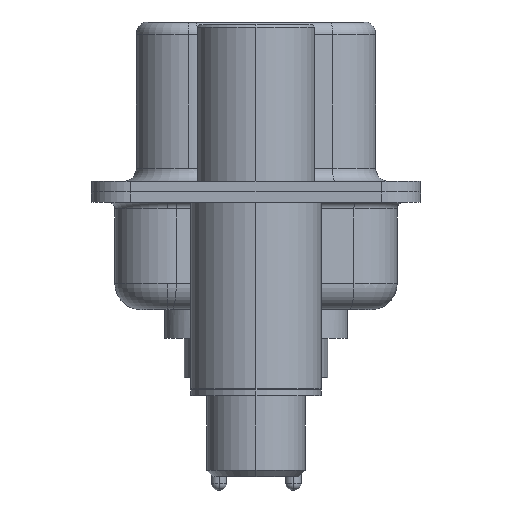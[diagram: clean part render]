
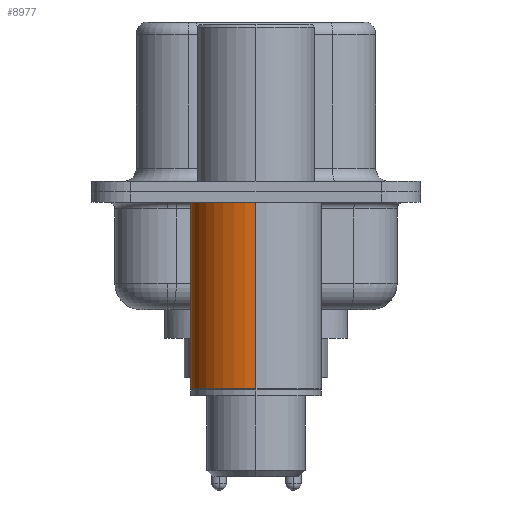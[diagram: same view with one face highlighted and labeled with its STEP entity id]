
A CAD part, left-side view. The second image highlights one B-rep face of the part: STEP entity #8977.
In plain terms, the highlighted cylindrical face has radius 2.5 mm (diameter 5 mm), a partial arc.
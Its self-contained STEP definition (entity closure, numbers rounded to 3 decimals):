
#102 = DIRECTION ( 'NONE',  ( 0., 0., 1. ) ) ;
#384 = CYLINDRICAL_SURFACE ( 'NONE', #8981, 2.5 ) ;
#977 = CARTESIAN_POINT ( 'NONE',  ( 2.5, 0., -0.4 ) ) ;
#1203 = DIRECTION ( 'NONE',  ( 1., 0., 0. ) ) ;
#2478 = EDGE_CURVE ( 'NONE', #8512, #4601, #16579, .T. ) ;
#2485 = ORIENTED_EDGE ( 'NONE', *, *, #2478, .F. ) ;
#2746 = DIRECTION ( 'NONE',  ( 0., 0., 1. ) ) ;
#3062 = DIRECTION ( 'NONE',  ( 0., 0., 1. ) ) ;
#3066 = LINE ( 'NONE', #19043, #12439 ) ;
#3137 = CARTESIAN_POINT ( 'NONE',  ( -2.5, 0., 0.581 ) ) ;
#3669 = EDGE_CURVE ( 'NONE', #4407, #8512, #3066, .T. ) ;
#3890 = AXIS2_PLACEMENT_3D ( 'NONE', #9927, #102, #1203 ) ;
#4407 = VERTEX_POINT ( 'NONE', #22356 ) ;
#4601 = VERTEX_POINT ( 'NONE', #20240 ) ;
#5339 = CIRCLE ( 'NONE', #20516, 2.5 ) ;
#5646 = FACE_OUTER_BOUND ( 'NONE', #13314, .T. ) ;
#6431 = DIRECTION ( 'NONE',  ( 0., 0., 1. ) ) ;
#6567 = ORIENTED_EDGE ( 'NONE', *, *, #9924, .T. ) ;
#7134 = ORIENTED_EDGE ( 'NONE', *, *, #3669, .F. ) ;
#8495 = CARTESIAN_POINT ( 'NONE',  ( -2.5, 0., -7.525 ) ) ;
#8512 = VERTEX_POINT ( 'NONE', #977 ) ;
#8977 = ADVANCED_FACE ( 'NONE', ( #5646 ), #384, .T. ) ;
#8981 = AXIS2_PLACEMENT_3D ( 'NONE', #14836, #6431, #10283 ) ;
#9924 = EDGE_CURVE ( 'NONE', #4407, #15791, #5339, .T. ) ;
#9927 = CARTESIAN_POINT ( 'NONE',  ( 0., 0., -0.4 ) ) ;
#10283 = DIRECTION ( 'NONE',  ( 1., 0., 0. ) ) ;
#10808 = DIRECTION ( 'NONE',  ( 0., 0., 1. ) ) ;
#11283 = ORIENTED_EDGE ( 'NONE', *, *, #18204, .T. ) ;
#12439 = VECTOR ( 'NONE', #10808, 1000. ) ;
#12789 = VECTOR ( 'NONE', #3062, 1000. ) ;
#13270 = CARTESIAN_POINT ( 'NONE',  ( 0., 0., -7.525 ) ) ;
#13314 = EDGE_LOOP ( 'NONE', ( #6567, #11283, #2485, #7134 ) ) ;
#13324 = LINE ( 'NONE', #3137, #12789 ) ;
#14836 = CARTESIAN_POINT ( 'NONE',  ( 0., 0., 0.581 ) ) ;
#15042 = DIRECTION ( 'NONE',  ( 1., 0., 0. ) ) ;
#15791 = VERTEX_POINT ( 'NONE', #8495 ) ;
#16579 = CIRCLE ( 'NONE', #3890, 2.5 ) ;
#18204 = EDGE_CURVE ( 'NONE', #15791, #4601, #13324, .T. ) ;
#19043 = CARTESIAN_POINT ( 'NONE',  ( 2.5, 0., 0.581 ) ) ;
#20240 = CARTESIAN_POINT ( 'NONE',  ( -2.5, 0., -0.4 ) ) ;
#20516 = AXIS2_PLACEMENT_3D ( 'NONE', #13270, #2746, #15042 ) ;
#22356 = CARTESIAN_POINT ( 'NONE',  ( 2.5, 0., -7.525 ) ) ;
